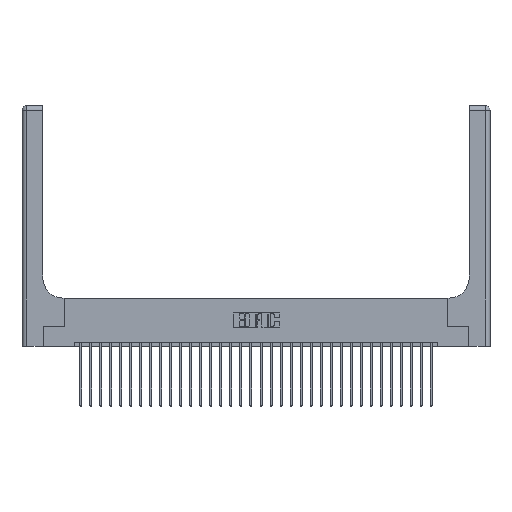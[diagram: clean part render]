
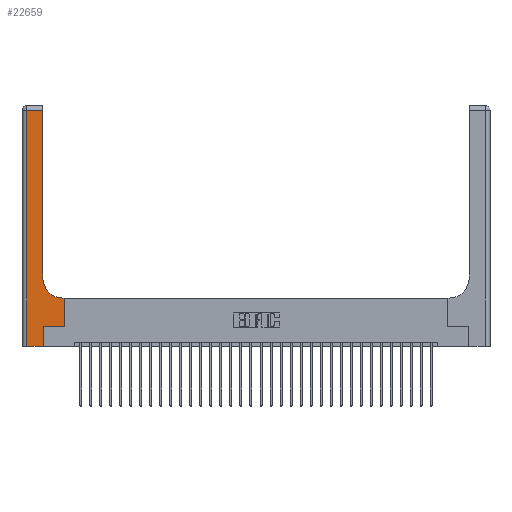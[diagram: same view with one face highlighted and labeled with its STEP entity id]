
A CAD part, top view. The second image highlights one B-rep face of the part: STEP entity #22659.
In plain terms, the highlighted planar face has unit normal (0, 0, 1).
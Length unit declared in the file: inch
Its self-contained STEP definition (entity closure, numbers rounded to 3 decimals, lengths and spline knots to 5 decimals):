
#510 = EDGE_CURVE ( 'NONE', #1166, #25584, #9041, .T. ) ;
#1166 = VERTEX_POINT ( 'NONE', #21790 ) ;
#1441 = CARTESIAN_POINT ( 'NONE',  ( 0.06, 2.94, 0.37 ) ) ;
#1761 = CARTESIAN_POINT ( 'NONE',  ( 0.51, 0.85, 0.37 ) ) ;
#1803 = LINE ( 'NONE', #13822, #12919 ) ;
#1839 = VERTEX_POINT ( 'NONE', #19261 ) ;
#1884 = FACE_OUTER_BOUND ( 'NONE', #8770, .T. ) ;
#2286 = ORIENTED_EDGE ( 'NONE', *, *, #15050, .T. ) ;
#3190 = ORIENTED_EDGE ( 'NONE', *, *, #18057, .T. ) ;
#3225 = VERTEX_POINT ( 'NONE', #22467 ) ;
#4011 = DIRECTION ( 'NONE',  ( -1., 0., 0. ) ) ;
#6039 = ORIENTED_EDGE ( 'NONE', *, *, #12366, .T. ) ;
#6235 = LINE ( 'NONE', #19165, #8410 ) ;
#6731 = VERTEX_POINT ( 'NONE', #12568 ) ;
#7395 = ORIENTED_EDGE ( 'NONE', *, *, #20278, .T. ) ;
#8410 = VECTOR ( 'NONE', #19062, 39.37008 ) ;
#8770 = EDGE_LOOP ( 'NONE', ( #20061, #14644, #6039, #17915, #11059, #2286, #27374, #7395, #3190 ) ) ;
#9041 = LINE ( 'NONE', #18597, #12261 ) ;
#9494 = DIRECTION ( 'NONE',  ( 0., 1., 0. ) ) ;
#9715 = VECTOR ( 'NONE', #9494, 39.37008 ) ;
#10159 = DIRECTION ( 'NONE',  ( 0., 1., 0. ) ) ;
#10349 = DIRECTION ( 'NONE',  ( -1., 0., 0. ) ) ;
#10675 = CARTESIAN_POINT ( 'NONE',  ( 0.528, 0.6, 0.37 ) ) ;
#11059 = ORIENTED_EDGE ( 'NONE', *, *, #23849, .T. ) ;
#11064 = CARTESIAN_POINT ( 'NONE',  ( 0., 3., 0.37 ) ) ;
#11363 = LINE ( 'NONE', #18187, #29155 ) ;
#11460 = LINE ( 'NONE', #18545, #9715 ) ;
#12227 = DIRECTION ( 'NONE',  ( 0., -1., 0. ) ) ;
#12261 = VECTOR ( 'NONE', #22175, 39.37008 ) ;
#12366 = EDGE_CURVE ( 'NONE', #25431, #6731, #1803, .T. ) ;
#12568 = CARTESIAN_POINT ( 'NONE',  ( 0.06, 0., 0.37 ) ) ;
#12639 = VERTEX_POINT ( 'NONE', #10675 ) ;
#12849 = VERTEX_POINT ( 'NONE', #21984 ) ;
#12919 = VECTOR ( 'NONE', #12227, 39.37008 ) ;
#13227 = VECTOR ( 'NONE', #10349, 39.37008 ) ;
#13605 = EDGE_CURVE ( 'NONE', #25584, #25431, #19263, .T. ) ;
#13822 = CARTESIAN_POINT ( 'NONE',  ( 0.06, 3., 0.37 ) ) ;
#14527 = CARTESIAN_POINT ( 'NONE',  ( 0.528, 0.25, 0.37 ) ) ;
#14644 = ORIENTED_EDGE ( 'NONE', *, *, #13605, .T. ) ;
#14966 = EDGE_CURVE ( 'NONE', #6731, #1839, #23383, .T. ) ;
#15050 = EDGE_CURVE ( 'NONE', #12849, #3225, #6235, .T. ) ;
#15180 = VERTEX_POINT ( 'NONE', #21958 ) ;
#15280 = DIRECTION ( 'NONE',  ( 1., 0., 0. ) ) ;
#15609 = AXIS2_PLACEMENT_3D ( 'NONE', #1761, #17726, #29158 ) ;
#15614 = DIRECTION ( 'NONE',  ( 0., 0., -1. ) ) ;
#16749 = LINE ( 'NONE', #14527, #22827 ) ;
#17476 = CARTESIAN_POINT ( 'NONE',  ( 0., 0., 0.37 ) ) ;
#17723 = PLANE ( 'NONE',  #26154 ) ;
#17726 = DIRECTION ( 'NONE',  ( 0., 0., -1. ) ) ;
#17915 = ORIENTED_EDGE ( 'NONE', *, *, #14966, .T. ) ;
#18057 = EDGE_CURVE ( 'NONE', #15180, #1166, #20013, .T. ) ;
#18187 = CARTESIAN_POINT ( 'NONE',  ( 0.26, 0.6, 0.37 ) ) ;
#18545 = CARTESIAN_POINT ( 'NONE',  ( 0.265, 0., 0.37 ) ) ;
#18597 = CARTESIAN_POINT ( 'NONE',  ( 0.26, 3., 0.37 ) ) ;
#19062 = DIRECTION ( 'NONE',  ( 1., 0., 0. ) ) ;
#19165 = CARTESIAN_POINT ( 'NONE',  ( 0.265, 0.25, 0.37 ) ) ;
#19204 = CARTESIAN_POINT ( 'NONE',  ( 0., 2.94, 0.37 ) ) ;
#19261 = CARTESIAN_POINT ( 'NONE',  ( 0.265, 0., 0.37 ) ) ;
#19263 = LINE ( 'NONE', #19204, #13227 ) ;
#20013 = CIRCLE ( 'NONE', #15609, 0.25 ) ;
#20061 = ORIENTED_EDGE ( 'NONE', *, *, #510, .T. ) ;
#20278 = EDGE_CURVE ( 'NONE', #12639, #15180, #11363, .T. ) ;
#21790 = CARTESIAN_POINT ( 'NONE',  ( 0.26, 0.85, 0.37 ) ) ;
#21958 = CARTESIAN_POINT ( 'NONE',  ( 0.51, 0.6, 0.37 ) ) ;
#21984 = CARTESIAN_POINT ( 'NONE',  ( 0.265, 0.25, 0.37 ) ) ;
#22175 = DIRECTION ( 'NONE',  ( 0., 1., 0. ) ) ;
#22467 = CARTESIAN_POINT ( 'NONE',  ( 0.528, 0.25, 0.37 ) ) ;
#22659 = ADVANCED_FACE ( 'NONE', ( #1884 ), #17723, .F. ) ;
#22827 = VECTOR ( 'NONE', #10159, 39.37008 ) ;
#23383 = LINE ( 'NONE', #17476, #24428 ) ;
#23849 = EDGE_CURVE ( 'NONE', #1839, #12849, #11460, .T. ) ;
#24428 = VECTOR ( 'NONE', #15280, 39.37008 ) ;
#24583 = CARTESIAN_POINT ( 'NONE',  ( 0.26, 2.94, 0.37 ) ) ;
#24718 = EDGE_CURVE ( 'NONE', #3225, #12639, #16749, .T. ) ;
#25431 = VERTEX_POINT ( 'NONE', #1441 ) ;
#25584 = VERTEX_POINT ( 'NONE', #24583 ) ;
#26154 = AXIS2_PLACEMENT_3D ( 'NONE', #11064, #15614, #4011 ) ;
#27314 = DIRECTION ( 'NONE',  ( -1., 0., 0. ) ) ;
#27374 = ORIENTED_EDGE ( 'NONE', *, *, #24718, .T. ) ;
#29155 = VECTOR ( 'NONE', #27314, 39.37008 ) ;
#29158 = DIRECTION ( 'NONE',  ( 1., 0., 0. ) ) ;
